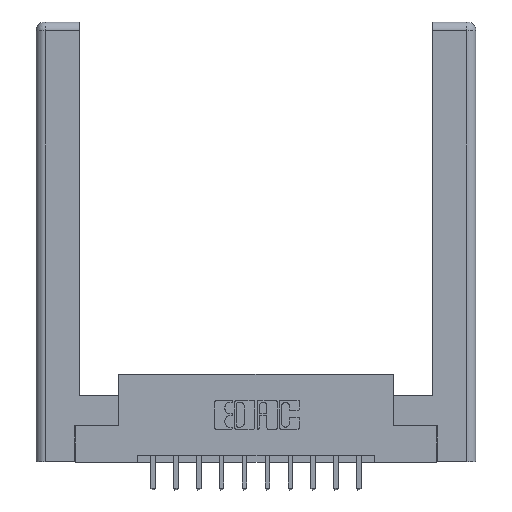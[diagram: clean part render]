
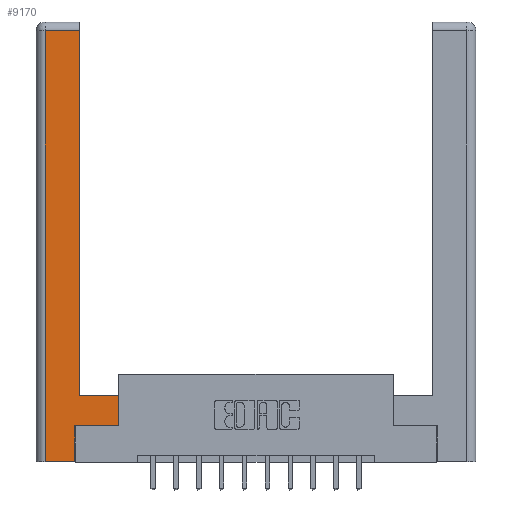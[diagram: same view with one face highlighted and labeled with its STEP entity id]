
A CAD part, top view. The second image highlights one B-rep face of the part: STEP entity #9170.
In plain terms, the highlighted planar face has unit normal (0, 0, 1).
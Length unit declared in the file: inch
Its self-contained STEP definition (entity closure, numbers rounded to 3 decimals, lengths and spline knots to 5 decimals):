
#1060 = CARTESIAN_POINT ( 'NONE',  ( 0.0615, 2.94, 0. ) ) ;
#1295 = ORIENTED_EDGE ( 'NONE', *, *, #11254, .T. ) ;
#1339 = ORIENTED_EDGE ( 'NONE', *, *, #5693, .T. ) ;
#1354 = CARTESIAN_POINT ( 'NONE',  ( 0.0615, 2.94, 0. ) ) ;
#1624 = VECTOR ( 'NONE', #3523, 39.37008 ) ;
#1732 = VECTOR ( 'NONE', #3165, 39.37008 ) ;
#1951 = DIRECTION ( 'NONE',  ( 0., 0., -1. ) ) ;
#1991 = LINE ( 'NONE', #11504, #6890 ) ;
#2016 = VECTOR ( 'NONE', #4236, 39.37008 ) ;
#2109 = ORIENTED_EDGE ( 'NONE', *, *, #12889, .T. ) ;
#2833 = VERTEX_POINT ( 'NONE', #4915 ) ;
#3014 = VECTOR ( 'NONE', #11865, 39.37008 ) ;
#3165 = DIRECTION ( 'NONE',  ( 0., 1., 0. ) ) ;
#3254 = EDGE_LOOP ( 'NONE', ( #9747, #6725, #2109, #4268, #1339, #4791, #4136, #1295 ) ) ;
#3523 = DIRECTION ( 'NONE',  ( 1., 0., 0. ) ) ;
#3707 = CARTESIAN_POINT ( 'NONE',  ( 0.295, 0.45, 0. ) ) ;
#3779 = CARTESIAN_POINT ( 'NONE',  ( 0.565, 0.245, 0. ) ) ;
#3966 = CARTESIAN_POINT ( 'NONE',  ( 0.295, 3., 0. ) ) ;
#4136 = ORIENTED_EDGE ( 'NONE', *, *, #10211, .T. ) ;
#4236 = DIRECTION ( 'NONE',  ( 0., -1., 0. ) ) ;
#4244 = CARTESIAN_POINT ( 'NONE',  ( 0., 0., 0. ) ) ;
#4268 = ORIENTED_EDGE ( 'NONE', *, *, #10118, .T. ) ;
#4363 = CARTESIAN_POINT ( 'NONE',  ( 0.565, 0.245, 0. ) ) ;
#4592 = LINE ( 'NONE', #1060, #6188 ) ;
#4647 = LINE ( 'NONE', #4363, #1624 ) ;
#4791 = ORIENTED_EDGE ( 'NONE', *, *, #6991, .T. ) ;
#4915 = CARTESIAN_POINT ( 'NONE',  ( 0.295, 2.94, 0. ) ) ;
#5398 = LINE ( 'NONE', #9919, #2016 ) ;
#5686 = VERTEX_POINT ( 'NONE', #3779 ) ;
#5689 = VERTEX_POINT ( 'NONE', #7906 ) ;
#5693 = EDGE_CURVE ( 'NONE', #12750, #5689, #8938, .T. ) ;
#5918 = VECTOR ( 'NONE', #13918, 39.37008 ) ;
#6188 = VECTOR ( 'NONE', #11441, 39.37008 ) ;
#6356 = LINE ( 'NONE', #8482, #7218 ) ;
#6725 = ORIENTED_EDGE ( 'NONE', *, *, #9386, .T. ) ;
#6890 = VECTOR ( 'NONE', #11739, 39.37008 ) ;
#6991 = EDGE_CURVE ( 'NONE', #5689, #5686, #4647, .T. ) ;
#7218 = VECTOR ( 'NONE', #10795, 39.37008 ) ;
#7532 = VERTEX_POINT ( 'NONE', #3707 ) ;
#7591 = PLANE ( 'NONE',  #10153 ) ;
#7906 = CARTESIAN_POINT ( 'NONE',  ( 0.265, 0.245, 0. ) ) ;
#8294 = CARTESIAN_POINT ( 'NONE',  ( 0.0615, 0., 0. ) ) ;
#8482 = CARTESIAN_POINT ( 'NONE',  ( 0.265, 0., 0. ) ) ;
#8938 = LINE ( 'NONE', #10348, #5918 ) ;
#9170 = ADVANCED_FACE ( 'NONE', ( #12216 ), #7591, .F. ) ;
#9386 = EDGE_CURVE ( 'NONE', #2833, #9994, #4592, .T. ) ;
#9434 = VERTEX_POINT ( 'NONE', #8294 ) ;
#9633 = EDGE_CURVE ( 'NONE', #7532, #2833, #9911, .T. ) ;
#9747 = ORIENTED_EDGE ( 'NONE', *, *, #9633, .T. ) ;
#9911 = LINE ( 'NONE', #3966, #3014 ) ;
#9919 = CARTESIAN_POINT ( 'NONE',  ( 0.0615, 0., 0. ) ) ;
#9994 = VERTEX_POINT ( 'NONE', #1354 ) ;
#10118 = EDGE_CURVE ( 'NONE', #9434, #12750, #6356, .T. ) ;
#10153 = AXIS2_PLACEMENT_3D ( 'NONE', #4244, #1951, #10988 ) ;
#10211 = EDGE_CURVE ( 'NONE', #5686, #12010, #11653, .T. ) ;
#10348 = CARTESIAN_POINT ( 'NONE',  ( 0.265, 0.245, 0. ) ) ;
#10795 = DIRECTION ( 'NONE',  ( 1., 0., 0. ) ) ;
#10988 = DIRECTION ( 'NONE',  ( -1., 0., 0. ) ) ;
#10989 = CARTESIAN_POINT ( 'NONE',  ( 0.565, 0.45, 0. ) ) ;
#11254 = EDGE_CURVE ( 'NONE', #12010, #7532, #1991, .T. ) ;
#11441 = DIRECTION ( 'NONE',  ( -1., 0., 0. ) ) ;
#11504 = CARTESIAN_POINT ( 'NONE',  ( 0.295, 0.45, 0. ) ) ;
#11653 = LINE ( 'NONE', #10989, #1732 ) ;
#11739 = DIRECTION ( 'NONE',  ( -1., 0., 0. ) ) ;
#11865 = DIRECTION ( 'NONE',  ( 0., 1., 0. ) ) ;
#11999 = CARTESIAN_POINT ( 'NONE',  ( 0.265, 0., 0. ) ) ;
#12010 = VERTEX_POINT ( 'NONE', #13614 ) ;
#12216 = FACE_OUTER_BOUND ( 'NONE', #3254, .T. ) ;
#12750 = VERTEX_POINT ( 'NONE', #11999 ) ;
#12889 = EDGE_CURVE ( 'NONE', #9994, #9434, #5398, .T. ) ;
#13614 = CARTESIAN_POINT ( 'NONE',  ( 0.565, 0.45, 0. ) ) ;
#13918 = DIRECTION ( 'NONE',  ( 0., 1., 0. ) ) ;
